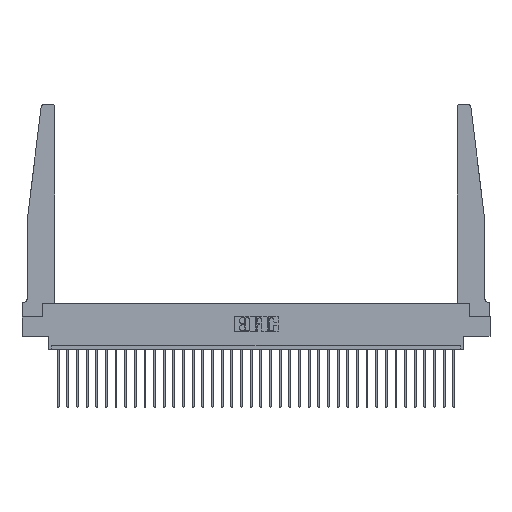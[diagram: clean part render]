
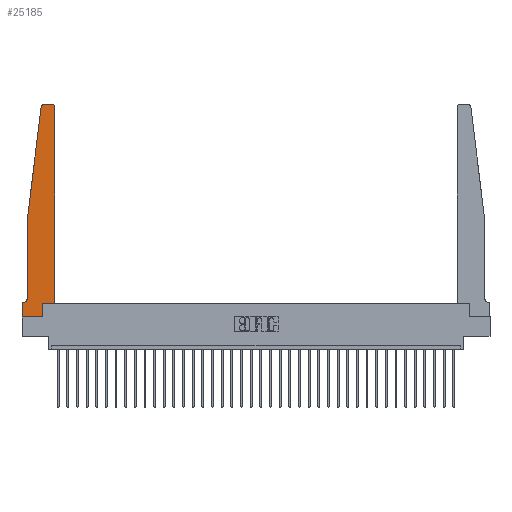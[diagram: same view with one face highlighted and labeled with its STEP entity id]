
A CAD part, top view. The second image highlights one B-rep face of the part: STEP entity #25185.
In plain terms, the highlighted planar face has unit normal (0, 0, 1).
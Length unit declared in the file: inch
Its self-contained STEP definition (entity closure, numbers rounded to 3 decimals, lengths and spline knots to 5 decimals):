
#366 = VECTOR ( 'NONE', #6855, 39.37008 ) ;
#485 = LINE ( 'NONE', #8532, #25215 ) ;
#736 = VERTEX_POINT ( 'NONE', #9184 ) ;
#1094 = AXIS2_PLACEMENT_3D ( 'NONE', #23736, #28925, #10056 ) ;
#1126 = AXIS2_PLACEMENT_3D ( 'NONE', #2415, #28760, #4830 ) ;
#1216 = DIRECTION ( 'NONE',  ( 1., 0., 0. ) ) ;
#1324 = LINE ( 'NONE', #30129, #8426 ) ;
#1332 = AXIS2_PLACEMENT_3D ( 'NONE', #23536, #16065, #13675 ) ;
#1353 = VERTEX_POINT ( 'NONE', #23702 ) ;
#1845 = LINE ( 'NONE', #5430, #26901 ) ;
#1956 = LINE ( 'NONE', #27013, #17245 ) ;
#2207 = LINE ( 'NONE', #10833, #19014 ) ;
#2415 = CARTESIAN_POINT ( 'NONE',  ( 0.015, 0.2375, 0.37 ) ) ;
#2426 = VECTOR ( 'NONE', #7628, 39.37008 ) ;
#2495 = FACE_OUTER_BOUND ( 'NONE', #7741, .T. ) ;
#2600 = DIRECTION ( 'NONE',  ( 0., 0., 1. ) ) ;
#2611 = VERTEX_POINT ( 'NONE', #18563 ) ;
#2932 = ORIENTED_EDGE ( 'NONE', *, *, #25596, .T. ) ;
#3448 = ORIENTED_EDGE ( 'NONE', *, *, #20709, .T. ) ;
#3532 = ORIENTED_EDGE ( 'NONE', *, *, #10387, .T. ) ;
#3549 = CARTESIAN_POINT ( 'NONE',  ( 0.25, 2.75, 0.37 ) ) ;
#4410 = AXIS2_PLACEMENT_3D ( 'NONE', #26132, #2600, #19290 ) ;
#4668 = CARTESIAN_POINT ( 'NONE',  ( 0.065, 0.2375, 0.37 ) ) ;
#4830 = DIRECTION ( 'NONE',  ( -1., 0., 0. ) ) ;
#4840 = CARTESIAN_POINT ( 'NONE',  ( 0.24675, 2.72367, 0.37 ) ) ;
#5430 = CARTESIAN_POINT ( 'NONE',  ( 0.065, 1.25, 0.37 ) ) ;
#5529 = DIRECTION ( 'NONE',  ( 0., -1., 0. ) ) ;
#6040 = CIRCLE ( 'NONE', #1094, 0.03 ) ;
#6685 = CARTESIAN_POINT ( 'NONE',  ( 0.395, 2.75, 0.37 ) ) ;
#6855 = DIRECTION ( 'NONE',  ( 0., -1., 0. ) ) ;
#7254 = CARTESIAN_POINT ( 'NONE',  ( 0.425, 0.18, 0.37 ) ) ;
#7458 = ORIENTED_EDGE ( 'NONE', *, *, #21893, .T. ) ;
#7628 = DIRECTION ( 'NONE',  ( 0., 1., 0. ) ) ;
#7741 = EDGE_LOOP ( 'NONE', ( #18550, #7458, #27277, #27064, #18783, #2932, #3532, #22663, #26355, #3448, #26622, #29748 ) ) ;
#7861 = EDGE_CURVE ( 'NONE', #19840, #19990, #8025, .T. ) ;
#8025 = LINE ( 'NONE', #20626, #27110 ) ;
#8426 = VECTOR ( 'NONE', #25441, 39.37008 ) ;
#8532 = CARTESIAN_POINT ( 'NONE',  ( 0.425, 0.18, 0.37 ) ) ;
#8903 = VERTEX_POINT ( 'NONE', #4668 ) ;
#9004 = VERTEX_POINT ( 'NONE', #29915 ) ;
#9184 = CARTESIAN_POINT ( 'NONE',  ( 0.27653, 2.75, 0.37 ) ) ;
#9376 = PLANE ( 'NONE',  #4410 ) ;
#10056 = DIRECTION ( 'NONE',  ( 1., 0., 0. ) ) ;
#10387 = EDGE_CURVE ( 'NONE', #20522, #2611, #25867, .T. ) ;
#10833 = CARTESIAN_POINT ( 'NONE',  ( 0.065, 1.25, 0.37 ) ) ;
#10972 = CARTESIAN_POINT ( 'NONE',  ( 0.425, 2.72, 0.37 ) ) ;
#11854 = CARTESIAN_POINT ( 'NONE',  ( 0., 0., 0.37 ) ) ;
#12337 = CARTESIAN_POINT ( 'NONE',  ( 0.425, 0.18, 0.37 ) ) ;
#12479 = VERTEX_POINT ( 'NONE', #6685 ) ;
#13675 = DIRECTION ( 'NONE',  ( 1., 0., 0. ) ) ;
#14201 = EDGE_CURVE ( 'NONE', #2611, #19840, #1956, .T. ) ;
#16065 = DIRECTION ( 'NONE',  ( 0., 0., 1. ) ) ;
#16184 = EDGE_CURVE ( 'NONE', #1353, #8903, #1845, .T. ) ;
#16485 = EDGE_CURVE ( 'NONE', #24768, #1353, #2207, .T. ) ;
#17245 = VECTOR ( 'NONE', #18018, 39.37008 ) ;
#17500 = DIRECTION ( 'NONE',  ( -1., 0., 0. ) ) ;
#17540 = CIRCLE ( 'NONE', #1332, 0.03 ) ;
#18018 = DIRECTION ( 'NONE',  ( 1., 0., 0. ) ) ;
#18550 = ORIENTED_EDGE ( 'NONE', *, *, #25355, .T. ) ;
#18563 = CARTESIAN_POINT ( 'NONE',  ( 0., 0., 0.37 ) ) ;
#18783 = ORIENTED_EDGE ( 'NONE', *, *, #28289, .T. ) ;
#19014 = VECTOR ( 'NONE', #20405, 39.37008 ) ;
#19290 = DIRECTION ( 'NONE',  ( 1., 0., 0. ) ) ;
#19391 = CIRCLE ( 'NONE', #1126, 0.05 ) ;
#19840 = VERTEX_POINT ( 'NONE', #21289 ) ;
#19990 = VERTEX_POINT ( 'NONE', #22688 ) ;
#20405 = DIRECTION ( 'NONE',  ( -0.122, -0.992, 0. ) ) ;
#20522 = VERTEX_POINT ( 'NONE', #21667 ) ;
#20626 = CARTESIAN_POINT ( 'NONE',  ( 0.2605, 0.18, 0.37 ) ) ;
#20709 = EDGE_CURVE ( 'NONE', #19990, #26962, #485, .T. ) ;
#21289 = CARTESIAN_POINT ( 'NONE',  ( 0.2605, 0., 0.37 ) ) ;
#21667 = CARTESIAN_POINT ( 'NONE',  ( 0., 0.1875, 0.37 ) ) ;
#21893 = EDGE_CURVE ( 'NONE', #736, #24768, #6040, .T. ) ;
#22663 = ORIENTED_EDGE ( 'NONE', *, *, #14201, .T. ) ;
#22688 = CARTESIAN_POINT ( 'NONE',  ( 0.2605, 0.18, 0.37 ) ) ;
#23500 = EDGE_CURVE ( 'NONE', #29792, #12479, #17540, .T. ) ;
#23536 = CARTESIAN_POINT ( 'NONE',  ( 0.395, 2.72, 0.37 ) ) ;
#23702 = CARTESIAN_POINT ( 'NONE',  ( 0.065, 1.25, 0.37 ) ) ;
#23736 = CARTESIAN_POINT ( 'NONE',  ( 0.27653, 2.72, 0.37 ) ) ;
#24538 = VECTOR ( 'NONE', #17500, 39.37008 ) ;
#24768 = VERTEX_POINT ( 'NONE', #4840 ) ;
#25185 = ADVANCED_FACE ( 'NONE', ( #2495 ), #9376, .T. ) ;
#25215 = VECTOR ( 'NONE', #1216, 39.37008 ) ;
#25242 = LINE ( 'NONE', #12337, #2426 ) ;
#25355 = EDGE_CURVE ( 'NONE', #12479, #736, #26765, .T. ) ;
#25441 = DIRECTION ( 'NONE',  ( -1., 0., 0. ) ) ;
#25596 = EDGE_CURVE ( 'NONE', #9004, #20522, #1324, .T. ) ;
#25867 = LINE ( 'NONE', #11854, #366 ) ;
#26132 = CARTESIAN_POINT ( 'NONE',  ( 0., 0.1875, 0.37 ) ) ;
#26188 = EDGE_CURVE ( 'NONE', #26962, #29792, #25242, .T. ) ;
#26355 = ORIENTED_EDGE ( 'NONE', *, *, #7861, .T. ) ;
#26622 = ORIENTED_EDGE ( 'NONE', *, *, #26188, .T. ) ;
#26765 = LINE ( 'NONE', #3549, #24538 ) ;
#26901 = VECTOR ( 'NONE', #5529, 39.37008 ) ;
#26962 = VERTEX_POINT ( 'NONE', #7254 ) ;
#27013 = CARTESIAN_POINT ( 'NONE',  ( 0., 0., 0.37 ) ) ;
#27064 = ORIENTED_EDGE ( 'NONE', *, *, #16184, .T. ) ;
#27110 = VECTOR ( 'NONE', #30632, 39.37008 ) ;
#27277 = ORIENTED_EDGE ( 'NONE', *, *, #16485, .T. ) ;
#28289 = EDGE_CURVE ( 'NONE', #8903, #9004, #19391, .T. ) ;
#28760 = DIRECTION ( 'NONE',  ( 0., 0., -1. ) ) ;
#28925 = DIRECTION ( 'NONE',  ( 0., 0., 1. ) ) ;
#29748 = ORIENTED_EDGE ( 'NONE', *, *, #23500, .T. ) ;
#29792 = VERTEX_POINT ( 'NONE', #10972 ) ;
#29915 = CARTESIAN_POINT ( 'NONE',  ( 0.015, 0.1875, 0.37 ) ) ;
#30129 = CARTESIAN_POINT ( 'NONE',  ( 0.065, 0.1875, 0.37 ) ) ;
#30632 = DIRECTION ( 'NONE',  ( 0., 1., 0. ) ) ;
